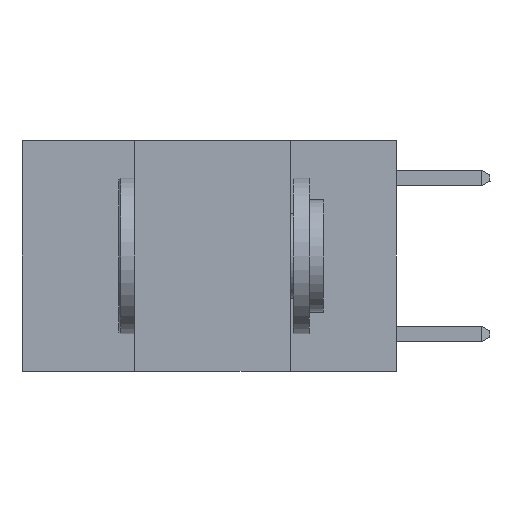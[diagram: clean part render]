
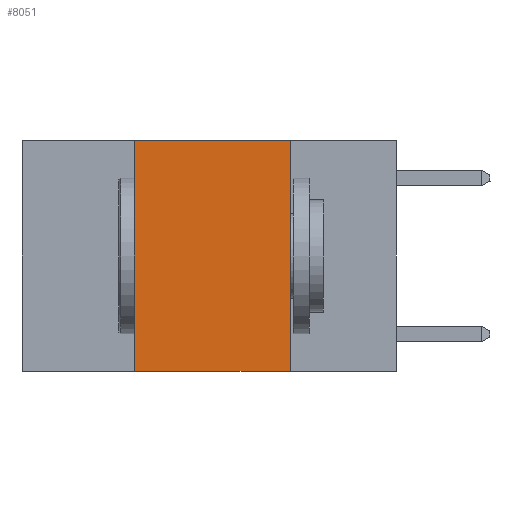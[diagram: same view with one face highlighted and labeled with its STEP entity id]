
A CAD part, left-side view. The second image highlights one B-rep face of the part: STEP entity #8051.
In plain terms, the highlighted planar face has unit normal (-1, 0, 0).
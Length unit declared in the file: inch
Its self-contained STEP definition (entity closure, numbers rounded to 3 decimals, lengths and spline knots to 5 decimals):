
#370 = CARTESIAN_POINT ( 'NONE',  ( 0., 0.6, 0. ) ) ;
#600 = LINE ( 'NONE', #8748, #7619 ) ;
#606 = CARTESIAN_POINT ( 'NONE',  ( 0., 0.17, -0.37 ) ) ;
#1717 = CARTESIAN_POINT ( 'NONE',  ( 0., 0.17, 0. ) ) ;
#2495 = PLANE ( 'NONE',  #2514 ) ;
#2514 = AXIS2_PLACEMENT_3D ( 'NONE', #370, #7386, #3198 ) ;
#2624 = CARTESIAN_POINT ( 'NONE',  ( 0., 0.6, 0. ) ) ;
#2714 = VERTEX_POINT ( 'NONE', #7533 ) ;
#2785 = LINE ( 'NONE', #6285, #6291 ) ;
#2819 = VERTEX_POINT ( 'NONE', #606 ) ;
#3198 = DIRECTION ( 'NONE',  ( 0., 0., -1. ) ) ;
#3845 = VERTEX_POINT ( 'NONE', #4961 ) ;
#4121 = ORIENTED_EDGE ( 'NONE', *, *, #4964, .F. ) ;
#4163 = EDGE_CURVE ( 'NONE', #2714, #7907, #600, .T. ) ;
#4308 = EDGE_CURVE ( 'NONE', #7907, #3845, #8363, .T. ) ;
#4401 = ORIENTED_EDGE ( 'NONE', *, *, #4163, .F. ) ;
#4733 = EDGE_CURVE ( 'NONE', #2714, #2819, #2785, .T. ) ;
#4869 = FACE_OUTER_BOUND ( 'NONE', #6295, .T. ) ;
#4961 = CARTESIAN_POINT ( 'NONE',  ( 0., 0.17, 0. ) ) ;
#4964 = EDGE_CURVE ( 'NONE', #3845, #2819, #8679, .T. ) ;
#5258 = DIRECTION ( 'NONE',  ( 0., 0., 1. ) ) ;
#5586 = DIRECTION ( 'NONE',  ( 0., -1., 0. ) ) ;
#5881 = ORIENTED_EDGE ( 'NONE', *, *, #4733, .T. ) ;
#6285 = CARTESIAN_POINT ( 'NONE',  ( 0., 0.6, -0.37 ) ) ;
#6291 = VECTOR ( 'NONE', #5586, 39.37008 ) ;
#6295 = EDGE_LOOP ( 'NONE', ( #4121, #7535, #4401, #5881 ) ) ;
#6613 = VECTOR ( 'NONE', #6623, 39.37008 ) ;
#6623 = DIRECTION ( 'NONE',  ( 0., 0., -1. ) ) ;
#6743 = VECTOR ( 'NONE', #7520, 39.37008 ) ;
#7180 = CARTESIAN_POINT ( 'NONE',  ( 0., 0.42, 0. ) ) ;
#7386 = DIRECTION ( 'NONE',  ( 1., 0., 0. ) ) ;
#7520 = DIRECTION ( 'NONE',  ( 0., -1., 0. ) ) ;
#7533 = CARTESIAN_POINT ( 'NONE',  ( 0., 0.42, -0.37 ) ) ;
#7535 = ORIENTED_EDGE ( 'NONE', *, *, #4308, .F. ) ;
#7619 = VECTOR ( 'NONE', #5258, 39.37008 ) ;
#7907 = VERTEX_POINT ( 'NONE', #7180 ) ;
#8051 = ADVANCED_FACE ( 'NONE', ( #4869 ), #2495, .F. ) ;
#8363 = LINE ( 'NONE', #2624, #6743 ) ;
#8679 = LINE ( 'NONE', #1717, #6613 ) ;
#8748 = CARTESIAN_POINT ( 'NONE',  ( 0., 0.42, 0. ) ) ;
